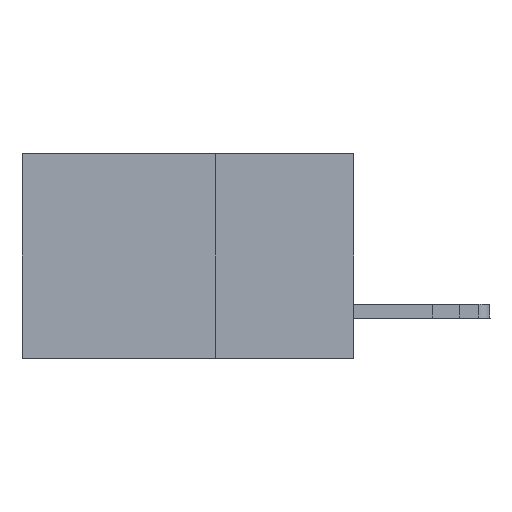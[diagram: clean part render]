
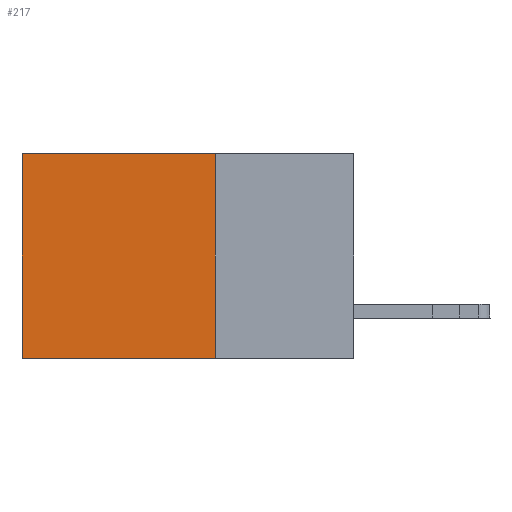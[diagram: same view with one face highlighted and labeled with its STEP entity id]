
A CAD part, left-side view. The second image highlights one B-rep face of the part: STEP entity #217.
In plain terms, the highlighted planar face has unit normal (-1, 0, 0).
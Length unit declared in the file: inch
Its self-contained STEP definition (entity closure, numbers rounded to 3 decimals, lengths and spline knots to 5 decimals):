
#217 = ADVANCED_FACE ( 'NONE', ( #2432 ), #7527, .F. ) ;
#969 = LINE ( 'NONE', #6461, #11149 ) ;
#1352 = CARTESIAN_POINT ( 'NONE',  ( 0.2875, 0.6, 0. ) ) ;
#1853 = EDGE_LOOP ( 'NONE', ( #3036, #21132, #16151, #16002 ) ) ;
#2305 = DIRECTION ( 'NONE',  ( 0., 0., -1. ) ) ;
#2332 = EDGE_CURVE ( 'NONE', #20676, #15141, #23808, .T. ) ;
#2432 = FACE_OUTER_BOUND ( 'NONE', #1853, .T. ) ;
#3036 = ORIENTED_EDGE ( 'NONE', *, *, #2332, .T. ) ;
#3149 = EDGE_CURVE ( 'NONE', #21642, #15141, #20577, .T. ) ;
#3381 = VERTEX_POINT ( 'NONE', #21887 ) ;
#5942 = DIRECTION ( 'NONE',  ( 0., 0., -1. ) ) ;
#6032 = CARTESIAN_POINT ( 'NONE',  ( 0.2875, 0.25, 0. ) ) ;
#6461 = CARTESIAN_POINT ( 'NONE',  ( 0.2875, 0.25, 0. ) ) ;
#7144 = CARTESIAN_POINT ( 'NONE',  ( 0.2875, 0.25, 0. ) ) ;
#7370 = DIRECTION ( 'NONE',  ( 1., 0., 0. ) ) ;
#7527 = PLANE ( 'NONE',  #10477 ) ;
#8590 = VECTOR ( 'NONE', #10729, 39.37008 ) ;
#10477 = AXIS2_PLACEMENT_3D ( 'NONE', #7144, #7370, #2305 ) ;
#10729 = DIRECTION ( 'NONE',  ( 0., 0., -1. ) ) ;
#10992 = VECTOR ( 'NONE', #13334, 39.37008 ) ;
#11149 = VECTOR ( 'NONE', #17948, 39.37008 ) ;
#11354 = CARTESIAN_POINT ( 'NONE',  ( 0.2875, 0.25, -0.37 ) ) ;
#12196 = VECTOR ( 'NONE', #5942, 39.37008 ) ;
#13334 = DIRECTION ( 'NONE',  ( 0., 1., 0. ) ) ;
#13963 = EDGE_CURVE ( 'NONE', #3381, #20676, #969, .T. ) ;
#14025 = CARTESIAN_POINT ( 'NONE',  ( 0.2875, 0.25, -0.37 ) ) ;
#15141 = VERTEX_POINT ( 'NONE', #19648 ) ;
#16002 = ORIENTED_EDGE ( 'NONE', *, *, #13963, .T. ) ;
#16151 = ORIENTED_EDGE ( 'NONE', *, *, #22712, .F. ) ;
#16512 = CARTESIAN_POINT ( 'NONE',  ( 0.2875, 0.6, 0. ) ) ;
#17948 = DIRECTION ( 'NONE',  ( 0., 1., 0. ) ) ;
#19648 = CARTESIAN_POINT ( 'NONE',  ( 0.2875, 0.6, -0.37 ) ) ;
#20577 = LINE ( 'NONE', #11354, #10992 ) ;
#20676 = VERTEX_POINT ( 'NONE', #1352 ) ;
#21132 = ORIENTED_EDGE ( 'NONE', *, *, #3149, .F. ) ;
#21642 = VERTEX_POINT ( 'NONE', #14025 ) ;
#21887 = CARTESIAN_POINT ( 'NONE',  ( 0.2875, 0.25, 0. ) ) ;
#22347 = LINE ( 'NONE', #6032, #12196 ) ;
#22712 = EDGE_CURVE ( 'NONE', #3381, #21642, #22347, .T. ) ;
#23808 = LINE ( 'NONE', #16512, #8590 ) ;
